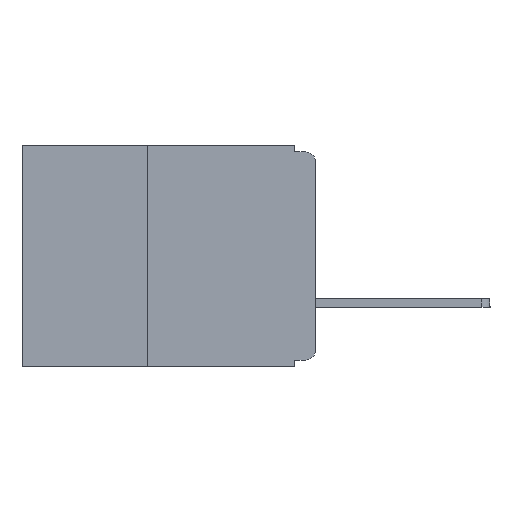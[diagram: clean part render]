
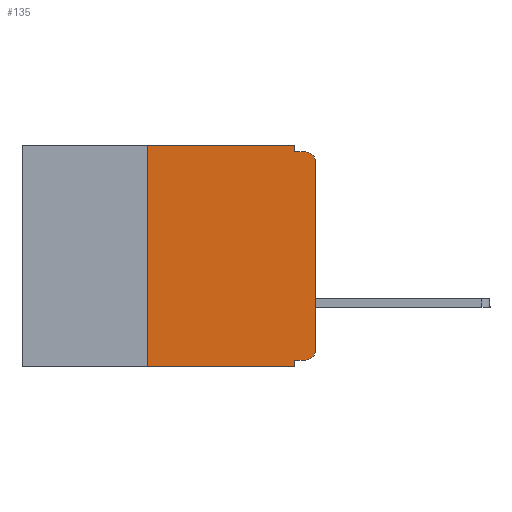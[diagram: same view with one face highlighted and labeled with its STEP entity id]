
A CAD part, left-side view. The second image highlights one B-rep face of the part: STEP entity #135.
In plain terms, the highlighted planar face has unit normal (-1, 0, 0).
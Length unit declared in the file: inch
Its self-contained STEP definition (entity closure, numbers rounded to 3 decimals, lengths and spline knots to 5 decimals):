
#135 = ADVANCED_FACE ( 'NONE', ( #14402 ), #18705, .F. ) ;
#649 = ORIENTED_EDGE ( 'NONE', *, *, #14884, .F. ) ;
#1272 = VERTEX_POINT ( 'NONE', #3884 ) ;
#1445 = CARTESIAN_POINT ( 'NONE',  ( 0., 0., -0.305 ) ) ;
#1571 = VECTOR ( 'NONE', #15131, 39.37008 ) ;
#1579 = ORIENTED_EDGE ( 'NONE', *, *, #13103, .F. ) ;
#2041 = CIRCLE ( 'NONE', #12317, 0.015 ) ;
#2650 = DIRECTION ( 'NONE',  ( 0., 0., 1. ) ) ;
#2959 = LINE ( 'NONE', #17231, #11739 ) ;
#3193 = EDGE_LOOP ( 'NONE', ( #11924, #7556, #11074, #1579, #9998, #11351, #8360, #649, #3208, #20482 ) ) ;
#3208 = ORIENTED_EDGE ( 'NONE', *, *, #18070, .F. ) ;
#3271 = DIRECTION ( 'NONE',  ( -1., 0., 0. ) ) ;
#3672 = EDGE_CURVE ( 'NONE', #15305, #1272, #9854, .T. ) ;
#3884 = CARTESIAN_POINT ( 'NONE',  ( 0., 0.031, -0.33 ) ) ;
#4013 = CARTESIAN_POINT ( 'NONE',  ( 0., 0.437, 0. ) ) ;
#4150 = DIRECTION ( 'NONE',  ( 1., 0., 0. ) ) ;
#4180 = DIRECTION ( 'NONE',  ( 0., 0., -1. ) ) ;
#4478 = CARTESIAN_POINT ( 'NONE',  ( 0., 0.015, -0.01 ) ) ;
#4489 = DIRECTION ( 'NONE',  ( 0., 0., -1. ) ) ;
#4664 = DIRECTION ( 'NONE',  ( 0., 1., 0. ) ) ;
#5139 = DIRECTION ( 'NONE',  ( -1., 0., 0. ) ) ;
#5163 = CIRCLE ( 'NONE', #14875, 0.015 ) ;
#5454 = DIRECTION ( 'NONE',  ( 0., 0., 1. ) ) ;
#5915 = VECTOR ( 'NONE', #5454, 39.37008 ) ;
#6061 = CARTESIAN_POINT ( 'NONE',  ( 0., 0.25, 0. ) ) ;
#6925 = VECTOR ( 'NONE', #4489, 39.37008 ) ;
#7214 = DIRECTION ( 'NONE',  ( 0., -1., 0. ) ) ;
#7319 = VERTEX_POINT ( 'NONE', #10468 ) ;
#7341 = DIRECTION ( 'NONE',  ( 0., 0., -1. ) ) ;
#7556 = ORIENTED_EDGE ( 'NONE', *, *, #20582, .T. ) ;
#8187 = LINE ( 'NONE', #9298, #20828 ) ;
#8360 = ORIENTED_EDGE ( 'NONE', *, *, #3672, .T. ) ;
#8704 = CARTESIAN_POINT ( 'NONE',  ( 0., 0.25, -0.33 ) ) ;
#9068 = LINE ( 'NONE', #18754, #17860 ) ;
#9105 = DIRECTION ( 'NONE',  ( 0., -1., 0. ) ) ;
#9272 = VERTEX_POINT ( 'NONE', #1445 ) ;
#9298 = CARTESIAN_POINT ( 'NONE',  ( 0., 0., 0. ) ) ;
#9854 = LINE ( 'NONE', #13443, #1571 ) ;
#9998 = ORIENTED_EDGE ( 'NONE', *, *, #11710, .F. ) ;
#10336 = LINE ( 'NONE', #13693, #5915 ) ;
#10468 = CARTESIAN_POINT ( 'NONE',  ( 0., 0.015, -0.32 ) ) ;
#11074 = ORIENTED_EDGE ( 'NONE', *, *, #17228, .F. ) ;
#11291 = CARTESIAN_POINT ( 'NONE',  ( 0., 0., -0.32 ) ) ;
#11296 = LINE ( 'NONE', #14298, #6925 ) ;
#11351 = ORIENTED_EDGE ( 'NONE', *, *, #17720, .F. ) ;
#11599 = VERTEX_POINT ( 'NONE', #15158 ) ;
#11625 = VERTEX_POINT ( 'NONE', #15233 ) ;
#11710 = EDGE_CURVE ( 'NONE', #13085, #13022, #9068, .T. ) ;
#11739 = VECTOR ( 'NONE', #7341, 39.37008 ) ;
#11885 = VECTOR ( 'NONE', #9105, 39.37008 ) ;
#11924 = ORIENTED_EDGE ( 'NONE', *, *, #13691, .T. ) ;
#12317 = AXIS2_PLACEMENT_3D ( 'NONE', #15041, #5139, #16697 ) ;
#12721 = EDGE_CURVE ( 'NONE', #7319, #9272, #2041, .T. ) ;
#12927 = AXIS2_PLACEMENT_3D ( 'NONE', #4013, #4150, #4180 ) ;
#13022 = VERTEX_POINT ( 'NONE', #15740 ) ;
#13085 = VERTEX_POINT ( 'NONE', #6061 ) ;
#13103 = EDGE_CURVE ( 'NONE', #13022, #11599, #11296, .T. ) ;
#13136 = CARTESIAN_POINT ( 'NONE',  ( 0., 0.015, -0.025 ) ) ;
#13443 = CARTESIAN_POINT ( 'NONE',  ( 0., 0.437, -0.33 ) ) ;
#13691 = EDGE_CURVE ( 'NONE', #9272, #20812, #8187, .T. ) ;
#13693 = CARTESIAN_POINT ( 'NONE',  ( 0., 0.25, -0.33 ) ) ;
#14298 = CARTESIAN_POINT ( 'NONE',  ( 0., 0.031, 0. ) ) ;
#14402 = FACE_OUTER_BOUND ( 'NONE', #3193, .T. ) ;
#14824 = DIRECTION ( 'NONE',  ( 0., 0., -1. ) ) ;
#14875 = AXIS2_PLACEMENT_3D ( 'NONE', #13136, #3271, #14824 ) ;
#14884 = EDGE_CURVE ( 'NONE', #11625, #1272, #2959, .T. ) ;
#15041 = CARTESIAN_POINT ( 'NONE',  ( 0., 0.015, -0.305 ) ) ;
#15131 = DIRECTION ( 'NONE',  ( 0., -1., 0. ) ) ;
#15158 = CARTESIAN_POINT ( 'NONE',  ( 0., 0.031, -0.01 ) ) ;
#15233 = CARTESIAN_POINT ( 'NONE',  ( 0., 0.031, -0.32 ) ) ;
#15305 = VERTEX_POINT ( 'NONE', #8704 ) ;
#15667 = CARTESIAN_POINT ( 'NONE',  ( 0., 0., -0.01 ) ) ;
#15740 = CARTESIAN_POINT ( 'NONE',  ( 0., 0.031, 0. ) ) ;
#16012 = VECTOR ( 'NONE', #4664, 39.37008 ) ;
#16189 = VERTEX_POINT ( 'NONE', #4478 ) ;
#16290 = LINE ( 'NONE', #15667, #11885 ) ;
#16697 = DIRECTION ( 'NONE',  ( 0., 0., -1. ) ) ;
#17228 = EDGE_CURVE ( 'NONE', #11599, #16189, #16290, .T. ) ;
#17231 = CARTESIAN_POINT ( 'NONE',  ( 0., 0.031, -0.33 ) ) ;
#17720 = EDGE_CURVE ( 'NONE', #15305, #13085, #10336, .T. ) ;
#17860 = VECTOR ( 'NONE', #7214, 39.37008 ) ;
#18070 = EDGE_CURVE ( 'NONE', #7319, #11625, #20915, .T. ) ;
#18705 = PLANE ( 'NONE',  #12927 ) ;
#18754 = CARTESIAN_POINT ( 'NONE',  ( 0., 0.437, 0. ) ) ;
#20352 = CARTESIAN_POINT ( 'NONE',  ( 0., 0., -0.025 ) ) ;
#20482 = ORIENTED_EDGE ( 'NONE', *, *, #12721, .T. ) ;
#20582 = EDGE_CURVE ( 'NONE', #20812, #16189, #5163, .T. ) ;
#20812 = VERTEX_POINT ( 'NONE', #20352 ) ;
#20828 = VECTOR ( 'NONE', #2650, 39.37008 ) ;
#20915 = LINE ( 'NONE', #11291, #16012 ) ;
